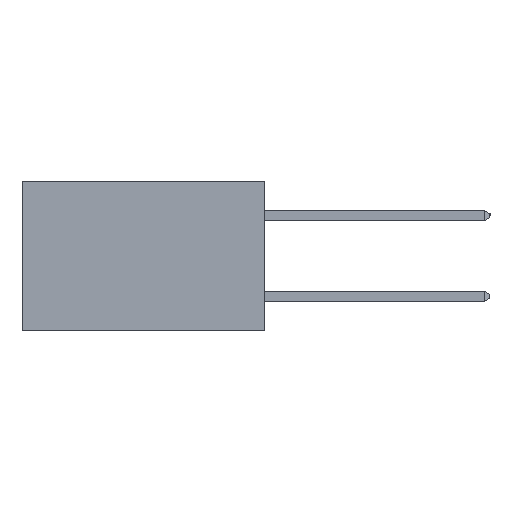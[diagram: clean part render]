
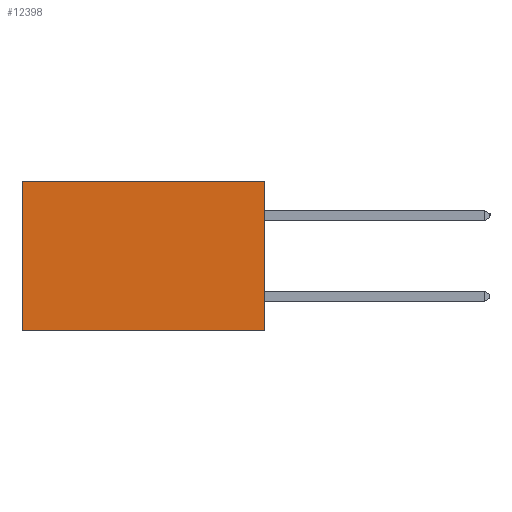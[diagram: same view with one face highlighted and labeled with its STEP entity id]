
A CAD part, left-side view. The second image highlights one B-rep face of the part: STEP entity #12398.
In plain terms, the highlighted planar face has unit normal (-1, 0, 0).
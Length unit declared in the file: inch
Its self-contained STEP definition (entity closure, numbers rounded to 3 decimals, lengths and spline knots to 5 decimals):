
#74 = DIRECTION ( 'NONE',  ( 0., 1., 0. ) ) ;
#444 = ORIENTED_EDGE ( 'NONE', *, *, #3651, .T. ) ;
#805 = CARTESIAN_POINT ( 'NONE',  ( 0.2615, 0.6, -0.37 ) ) ;
#1783 = CARTESIAN_POINT ( 'NONE',  ( 0.2615, 0.6, 0. ) ) ;
#2509 = VECTOR ( 'NONE', #16815, 39.37008 ) ;
#2628 = VERTEX_POINT ( 'NONE', #805 ) ;
#3345 = EDGE_CURVE ( 'NONE', #4960, #2628, #19418, .T. ) ;
#3651 = EDGE_CURVE ( 'NONE', #16568, #4960, #20937, .T. ) ;
#4942 = EDGE_CURVE ( 'NONE', #16568, #21161, #5163, .T. ) ;
#4960 = VERTEX_POINT ( 'NONE', #1783 ) ;
#5163 = LINE ( 'NONE', #18955, #20737 ) ;
#6257 = EDGE_CURVE ( 'NONE', #21161, #2628, #17034, .T. ) ;
#6273 = CARTESIAN_POINT ( 'NONE',  ( 0.2615, 0.6, -0.37 ) ) ;
#7324 = ORIENTED_EDGE ( 'NONE', *, *, #4942, .F. ) ;
#8894 = VECTOR ( 'NONE', #74, 39.37008 ) ;
#10249 = AXIS2_PLACEMENT_3D ( 'NONE', #17250, #18804, #19053 ) ;
#11542 = ORIENTED_EDGE ( 'NONE', *, *, #3345, .T. ) ;
#11979 = CARTESIAN_POINT ( 'NONE',  ( 0.2615, 0., -0.37 ) ) ;
#12246 = FACE_OUTER_BOUND ( 'NONE', #16080, .T. ) ;
#12398 = ADVANCED_FACE ( 'NONE', ( #12246 ), #20370, .F. ) ;
#14313 = ORIENTED_EDGE ( 'NONE', *, *, #6257, .F. ) ;
#15232 = CARTESIAN_POINT ( 'NONE',  ( 0.2615, 0., -0.37 ) ) ;
#15725 = CARTESIAN_POINT ( 'NONE',  ( 0.2615, 0., 0. ) ) ;
#16080 = EDGE_LOOP ( 'NONE', ( #11542, #14313, #7324, #444 ) ) ;
#16568 = VERTEX_POINT ( 'NONE', #15725 ) ;
#16815 = DIRECTION ( 'NONE',  ( 0., 1., 0. ) ) ;
#17034 = LINE ( 'NONE', #15232, #2509 ) ;
#17250 = CARTESIAN_POINT ( 'NONE',  ( 0.2615, 0., -0.37 ) ) ;
#17582 = CARTESIAN_POINT ( 'NONE',  ( 0.2615, 0., 0. ) ) ;
#17734 = DIRECTION ( 'NONE',  ( 0., 0., -1. ) ) ;
#17831 = VECTOR ( 'NONE', #17734, 39.37008 ) ;
#18722 = DIRECTION ( 'NONE',  ( 0., 0., -1. ) ) ;
#18804 = DIRECTION ( 'NONE',  ( 1., 0., 0. ) ) ;
#18955 = CARTESIAN_POINT ( 'NONE',  ( 0.2615, 0., -0.37 ) ) ;
#19053 = DIRECTION ( 'NONE',  ( 0., 0., -1. ) ) ;
#19418 = LINE ( 'NONE', #6273, #17831 ) ;
#20370 = PLANE ( 'NONE',  #10249 ) ;
#20737 = VECTOR ( 'NONE', #18722, 39.37008 ) ;
#20937 = LINE ( 'NONE', #17582, #8894 ) ;
#21161 = VERTEX_POINT ( 'NONE', #11979 ) ;
